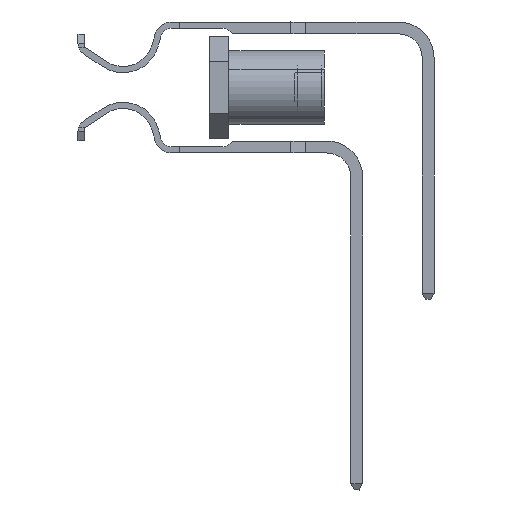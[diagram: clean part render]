
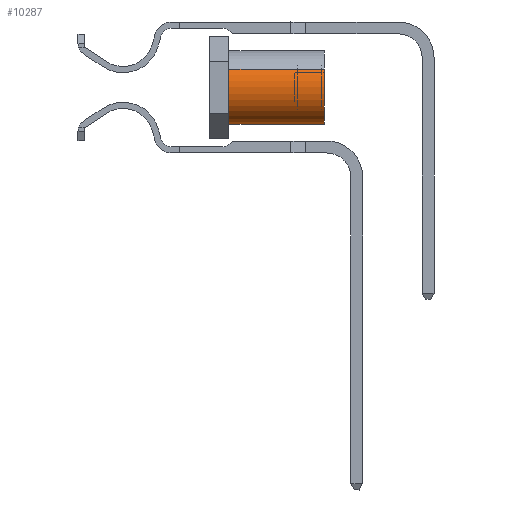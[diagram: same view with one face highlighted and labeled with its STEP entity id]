
A CAD part, left-side view. The second image highlights one B-rep face of the part: STEP entity #10287.
In plain terms, the highlighted cylindrical face has radius 1.968 mm (diameter 3.937 mm), a partial arc.
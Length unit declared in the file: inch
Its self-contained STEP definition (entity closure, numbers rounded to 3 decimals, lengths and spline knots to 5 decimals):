
#232 = VECTOR ( 'NONE', #12144, 39.37008 ) ;
#521 = DIRECTION ( 'NONE',  ( 0., 1., 0. ) ) ;
#1344 = CARTESIAN_POINT ( 'NONE',  ( 0., 0.24, 0. ) ) ;
#2080 = CARTESIAN_POINT ( 'NONE',  ( 0., 0.24, -0.0775 ) ) ;
#2273 = AXIS2_PLACEMENT_3D ( 'NONE', #12527, #521, #14524 ) ;
#2315 = VERTEX_POINT ( 'NONE', #15399 ) ;
#2371 = CARTESIAN_POINT ( 'NONE',  ( 0., 0.24, 0.0775 ) ) ;
#2506 = VERTEX_POINT ( 'NONE', #8027 ) ;
#2699 = EDGE_CURVE ( 'NONE', #5596, #14516, #6465, .T. ) ;
#3371 = EDGE_LOOP ( 'NONE', ( #25620, #11048, #19758, #25282 ) ) ;
#3853 = VECTOR ( 'NONE', #12337, 39.37008 ) ;
#4673 = CYLINDRICAL_SURFACE ( 'NONE', #14101, 0.0775 ) ;
#4854 = DIRECTION ( 'NONE',  ( 0., 1., 0. ) ) ;
#5596 = VERTEX_POINT ( 'NONE', #20563 ) ;
#6465 = CIRCLE ( 'NONE', #2273, 0.0775 ) ;
#8027 = CARTESIAN_POINT ( 'NONE',  ( 0., 0.04, 0.0775 ) ) ;
#10287 = ADVANCED_FACE ( 'NONE', ( #25745 ), #4673, .T. ) ;
#11048 = ORIENTED_EDGE ( 'NONE', *, *, #2699, .F. ) ;
#12144 = DIRECTION ( 'NONE',  ( 0., -1., 0. ) ) ;
#12218 = CARTESIAN_POINT ( 'NONE',  ( 0., 0.24, 0.0775 ) ) ;
#12337 = DIRECTION ( 'NONE',  ( 0., -1., 0. ) ) ;
#12527 = CARTESIAN_POINT ( 'NONE',  ( 0., 0.24, 0. ) ) ;
#13816 = LINE ( 'NONE', #2371, #3853 ) ;
#13893 = EDGE_CURVE ( 'NONE', #14516, #2506, #13816, .T. ) ;
#14101 = AXIS2_PLACEMENT_3D ( 'NONE', #1344, #17331, #15252 ) ;
#14516 = VERTEX_POINT ( 'NONE', #12218 ) ;
#14524 = DIRECTION ( 'NONE',  ( 0., 0., 1. ) ) ;
#15252 = DIRECTION ( 'NONE',  ( 0., 0., -1. ) ) ;
#15399 = CARTESIAN_POINT ( 'NONE',  ( 0., 0.04, -0.0775 ) ) ;
#16060 = EDGE_CURVE ( 'NONE', #5596, #2315, #16183, .T. ) ;
#16183 = LINE ( 'NONE', #2080, #232 ) ;
#16773 = CARTESIAN_POINT ( 'NONE',  ( 0., 0.04, 0. ) ) ;
#17331 = DIRECTION ( 'NONE',  ( 0., -1., 0. ) ) ;
#18749 = DIRECTION ( 'NONE',  ( 0., 0., 1. ) ) ;
#19758 = ORIENTED_EDGE ( 'NONE', *, *, #16060, .T. ) ;
#20563 = CARTESIAN_POINT ( 'NONE',  ( 0., 0.24, -0.0775 ) ) ;
#21998 = CIRCLE ( 'NONE', #25202, 0.0775 ) ;
#23623 = EDGE_CURVE ( 'NONE', #2315, #2506, #21998, .T. ) ;
#25202 = AXIS2_PLACEMENT_3D ( 'NONE', #16773, #4854, #18749 ) ;
#25282 = ORIENTED_EDGE ( 'NONE', *, *, #23623, .T. ) ;
#25620 = ORIENTED_EDGE ( 'NONE', *, *, #13893, .F. ) ;
#25745 = FACE_OUTER_BOUND ( 'NONE', #3371, .T. ) ;
